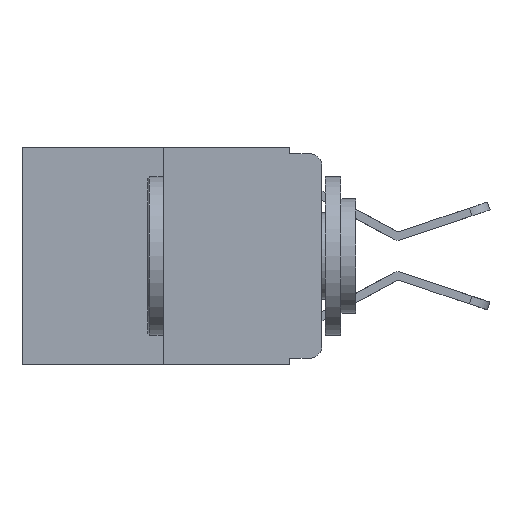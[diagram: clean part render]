
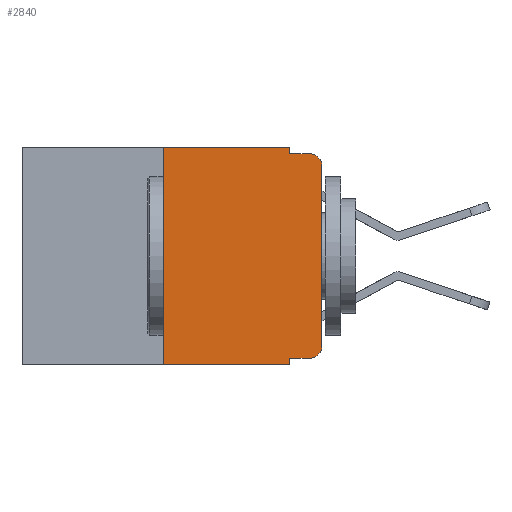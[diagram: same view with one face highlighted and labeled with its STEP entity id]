
A CAD part, left-side view. The second image highlights one B-rep face of the part: STEP entity #2840.
In plain terms, the highlighted planar face has unit normal (-1, 0, 0).
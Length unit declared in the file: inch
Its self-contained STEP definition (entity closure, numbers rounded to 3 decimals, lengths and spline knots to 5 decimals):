
#747 = DIRECTION ( 'NONE',  ( 0., -1., 0. ) ) ;
#1339 = VERTEX_POINT ( 'NONE', #4018 ) ;
#1348 = VERTEX_POINT ( 'NONE', #10877 ) ;
#1410 = CARTESIAN_POINT ( 'NONE',  ( 0., 0.02, -0.313 ) ) ;
#1420 = CARTESIAN_POINT ( 'NONE',  ( 0., 0.473, 0. ) ) ;
#1486 = ORIENTED_EDGE ( 'NONE', *, *, #13563, .T. ) ;
#1666 = VERTEX_POINT ( 'NONE', #14670 ) ;
#1868 = EDGE_CURVE ( 'NONE', #5826, #1348, #5206, .T. ) ;
#2022 = VECTOR ( 'NONE', #9984, 39.37008 ) ;
#2605 = DIRECTION ( 'NONE',  ( 0., 0., -1. ) ) ;
#2614 = DIRECTION ( 'NONE',  ( 0., -1., 0. ) ) ;
#2672 = EDGE_CURVE ( 'NONE', #1666, #1339, #12512, .T. ) ;
#2769 = ORIENTED_EDGE ( 'NONE', *, *, #1868, .F. ) ;
#2826 = VERTEX_POINT ( 'NONE', #13102 ) ;
#2840 = ADVANCED_FACE ( 'NONE', ( #4060 ), #8600, .F. ) ;
#2860 = AXIS2_PLACEMENT_3D ( 'NONE', #10109, #10161, #7693 ) ;
#3077 = LINE ( 'NONE', #1420, #14702 ) ;
#3127 = CARTESIAN_POINT ( 'NONE',  ( 0., 0.473, -0.343 ) ) ;
#3462 = EDGE_CURVE ( 'NONE', #9401, #7883, #13573, .T. ) ;
#3490 = VECTOR ( 'NONE', #6556, 39.37008 ) ;
#4018 = CARTESIAN_POINT ( 'NONE',  ( 0., 0.25, 0. ) ) ;
#4036 = LINE ( 'NONE', #8936, #10456 ) ;
#4060 = FACE_OUTER_BOUND ( 'NONE', #6325, .T. ) ;
#4257 = CARTESIAN_POINT ( 'NONE',  ( 0., 0.051, -0.01 ) ) ;
#4555 = CARTESIAN_POINT ( 'NONE',  ( 0., 0.051, -0.333 ) ) ;
#4636 = VECTOR ( 'NONE', #10015, 39.37008 ) ;
#4678 = VECTOR ( 'NONE', #5967, 39.37008 ) ;
#4809 = VECTOR ( 'NONE', #11022, 39.37008 ) ;
#5095 = EDGE_CURVE ( 'NONE', #7883, #5293, #13701, .T. ) ;
#5206 = LINE ( 'NONE', #8972, #2022 ) ;
#5293 = VERTEX_POINT ( 'NONE', #6940 ) ;
#5532 = ORIENTED_EDGE ( 'NONE', *, *, #2672, .F. ) ;
#5665 = VECTOR ( 'NONE', #747, 39.37008 ) ;
#5711 = ORIENTED_EDGE ( 'NONE', *, *, #5095, .F. ) ;
#5826 = VERTEX_POINT ( 'NONE', #4555 ) ;
#5967 = DIRECTION ( 'NONE',  ( 0., 0., -1. ) ) ;
#6019 = CARTESIAN_POINT ( 'NONE',  ( 0., 0.02, -0.03 ) ) ;
#6083 = EDGE_CURVE ( 'NONE', #1339, #9401, #3077, .T. ) ;
#6234 = CIRCLE ( 'NONE', #10003, 0.02 ) ;
#6295 = ORIENTED_EDGE ( 'NONE', *, *, #14283, .T. ) ;
#6325 = EDGE_LOOP ( 'NONE', ( #10288, #11301, #5711, #8720, #13356, #5532, #12530, #2769, #6295, #1486 ) ) ;
#6556 = DIRECTION ( 'NONE',  ( 0., 0., 1. ) ) ;
#6609 = EDGE_CURVE ( 'NONE', #7815, #5293, #8468, .T. ) ;
#6828 = CARTESIAN_POINT ( 'NONE',  ( 0., 0.25, 0. ) ) ;
#6839 = CARTESIAN_POINT ( 'NONE',  ( 0., 0.051, 0. ) ) ;
#6940 = CARTESIAN_POINT ( 'NONE',  ( 0., 0.02, -0.01 ) ) ;
#7006 = CARTESIAN_POINT ( 'NONE',  ( 0., 0.051, 0. ) ) ;
#7160 = DIRECTION ( 'NONE',  ( 0., 0., -1. ) ) ;
#7693 = DIRECTION ( 'NONE',  ( 0., 0., -1. ) ) ;
#7815 = VERTEX_POINT ( 'NONE', #10935 ) ;
#7883 = VERTEX_POINT ( 'NONE', #12215 ) ;
#7980 = AXIS2_PLACEMENT_3D ( 'NONE', #6019, #13764, #7160 ) ;
#8468 = CIRCLE ( 'NONE', #7980, 0.02 ) ;
#8600 = PLANE ( 'NONE',  #2860 ) ;
#8720 = ORIENTED_EDGE ( 'NONE', *, *, #3462, .F. ) ;
#8936 = CARTESIAN_POINT ( 'NONE',  ( 0., 0., 0. ) ) ;
#8972 = CARTESIAN_POINT ( 'NONE',  ( 0., 0.051, 0. ) ) ;
#9401 = VERTEX_POINT ( 'NONE', #6839 ) ;
#9527 = DIRECTION ( 'NONE',  ( -1., 0., 0. ) ) ;
#9642 = EDGE_CURVE ( 'NONE', #12892, #7815, #4036, .T. ) ;
#9984 = DIRECTION ( 'NONE',  ( 0., 0., -1. ) ) ;
#10003 = AXIS2_PLACEMENT_3D ( 'NONE', #1410, #9527, #2605 ) ;
#10015 = DIRECTION ( 'NONE',  ( 0., -1., 0. ) ) ;
#10109 = CARTESIAN_POINT ( 'NONE',  ( 0., 0.473, 0. ) ) ;
#10161 = DIRECTION ( 'NONE',  ( 1., 0., 0. ) ) ;
#10288 = ORIENTED_EDGE ( 'NONE', *, *, #9642, .T. ) ;
#10456 = VECTOR ( 'NONE', #11096, 39.37008 ) ;
#10877 = CARTESIAN_POINT ( 'NONE',  ( 0., 0.051, -0.343 ) ) ;
#10935 = CARTESIAN_POINT ( 'NONE',  ( 0., 0., -0.03 ) ) ;
#11022 = DIRECTION ( 'NONE',  ( 0., -1., 0. ) ) ;
#11096 = DIRECTION ( 'NONE',  ( 0., 0., 1. ) ) ;
#11258 = LINE ( 'NONE', #14358, #5665 ) ;
#11301 = ORIENTED_EDGE ( 'NONE', *, *, #6609, .T. ) ;
#12215 = CARTESIAN_POINT ( 'NONE',  ( 0., 0.051, -0.01 ) ) ;
#12512 = LINE ( 'NONE', #6828, #3490 ) ;
#12530 = ORIENTED_EDGE ( 'NONE', *, *, #12679, .T. ) ;
#12679 = EDGE_CURVE ( 'NONE', #1666, #1348, #13195, .T. ) ;
#12892 = VERTEX_POINT ( 'NONE', #13643 ) ;
#13102 = CARTESIAN_POINT ( 'NONE',  ( 0., 0.02, -0.333 ) ) ;
#13195 = LINE ( 'NONE', #3127, #4636 ) ;
#13356 = ORIENTED_EDGE ( 'NONE', *, *, #6083, .F. ) ;
#13563 = EDGE_CURVE ( 'NONE', #2826, #12892, #6234, .T. ) ;
#13573 = LINE ( 'NONE', #7006, #4678 ) ;
#13643 = CARTESIAN_POINT ( 'NONE',  ( 0., 0., -0.313 ) ) ;
#13701 = LINE ( 'NONE', #4257, #4809 ) ;
#13764 = DIRECTION ( 'NONE',  ( -1., 0., 0. ) ) ;
#14283 = EDGE_CURVE ( 'NONE', #5826, #2826, #11258, .T. ) ;
#14358 = CARTESIAN_POINT ( 'NONE',  ( 0., 0.051, -0.333 ) ) ;
#14670 = CARTESIAN_POINT ( 'NONE',  ( 0., 0.25, -0.343 ) ) ;
#14702 = VECTOR ( 'NONE', #2614, 39.37008 ) ;
